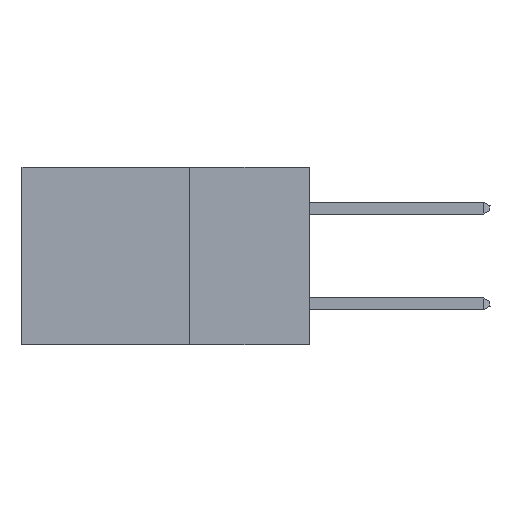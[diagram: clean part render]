
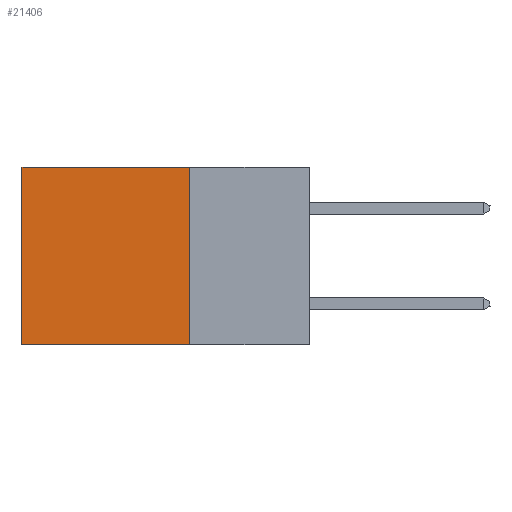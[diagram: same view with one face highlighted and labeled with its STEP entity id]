
A CAD part, left-side view. The second image highlights one B-rep face of the part: STEP entity #21406.
In plain terms, the highlighted planar face has unit normal (-1, 0, 0).
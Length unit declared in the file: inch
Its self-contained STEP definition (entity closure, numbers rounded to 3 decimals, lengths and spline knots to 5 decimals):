
#2016 = DIRECTION ( 'NONE',  ( 0., 0., -1. ) ) ;
#3122 = EDGE_LOOP ( 'NONE', ( #9789, #17214, #21053, #15504 ) ) ;
#6046 = VERTEX_POINT ( 'NONE', #35560 ) ;
#6165 = EDGE_CURVE ( 'NONE', #33229, #18951, #35099, .T. ) ;
#8092 = VECTOR ( 'NONE', #9050, 39.37008 ) ;
#9050 = DIRECTION ( 'NONE',  ( 0., 1., 0. ) ) ;
#9183 = CARTESIAN_POINT ( 'NONE',  ( 0.2875, 0.25, 0. ) ) ;
#9653 = FACE_OUTER_BOUND ( 'NONE', #3122, .T. ) ;
#9789 = ORIENTED_EDGE ( 'NONE', *, *, #24479, .T. ) ;
#9841 = VECTOR ( 'NONE', #18636, 39.37008 ) ;
#10982 = CARTESIAN_POINT ( 'NONE',  ( 0.2875, 0.25, 0. ) ) ;
#15504 = ORIENTED_EDGE ( 'NONE', *, *, #36064, .T. ) ;
#16427 = PLANE ( 'NONE',  #23688 ) ;
#16821 = VECTOR ( 'NONE', #26266, 39.37008 ) ;
#17214 = ORIENTED_EDGE ( 'NONE', *, *, #36032, .F. ) ;
#18260 = CARTESIAN_POINT ( 'NONE',  ( 0.2875, 0.6, 0. ) ) ;
#18636 = DIRECTION ( 'NONE',  ( 0., 0., -1. ) ) ;
#18951 = VERTEX_POINT ( 'NONE', #25800 ) ;
#19236 = DIRECTION ( 'NONE',  ( 0., 0., -1. ) ) ;
#19801 = CARTESIAN_POINT ( 'NONE',  ( 0.2875, 0.25, 0. ) ) ;
#21053 = ORIENTED_EDGE ( 'NONE', *, *, #6165, .F. ) ;
#21137 = CARTESIAN_POINT ( 'NONE',  ( 0.2875, 0.6, -0.37 ) ) ;
#21406 = ADVANCED_FACE ( 'NONE', ( #9653 ), #16427, .F. ) ;
#23688 = AXIS2_PLACEMENT_3D ( 'NONE', #28525, #25665, #19236 ) ;
#24124 = LINE ( 'NONE', #18260, #9841 ) ;
#24479 = EDGE_CURVE ( 'NONE', #6046, #32959, #24124, .T. ) ;
#25665 = DIRECTION ( 'NONE',  ( 1., 0., 0. ) ) ;
#25800 = CARTESIAN_POINT ( 'NONE',  ( 0.2875, 0.25, -0.37 ) ) ;
#26251 = VECTOR ( 'NONE', #2016, 39.37008 ) ;
#26266 = DIRECTION ( 'NONE',  ( 0., 1., 0. ) ) ;
#27421 = LINE ( 'NONE', #32501, #8092 ) ;
#28525 = CARTESIAN_POINT ( 'NONE',  ( 0.2875, 0.25, 0. ) ) ;
#32501 = CARTESIAN_POINT ( 'NONE',  ( 0.2875, 0.25, -0.37 ) ) ;
#32959 = VERTEX_POINT ( 'NONE', #21137 ) ;
#33229 = VERTEX_POINT ( 'NONE', #19801 ) ;
#35099 = LINE ( 'NONE', #10982, #26251 ) ;
#35560 = CARTESIAN_POINT ( 'NONE',  ( 0.2875, 0.6, 0. ) ) ;
#36032 = EDGE_CURVE ( 'NONE', #18951, #32959, #27421, .T. ) ;
#36064 = EDGE_CURVE ( 'NONE', #33229, #6046, #36221, .T. ) ;
#36221 = LINE ( 'NONE', #9183, #16821 ) ;
